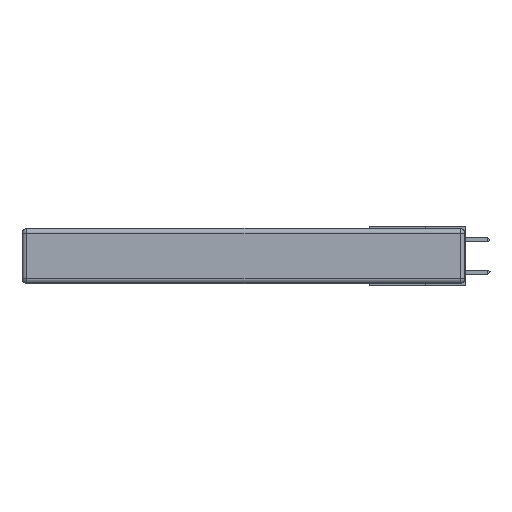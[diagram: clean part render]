
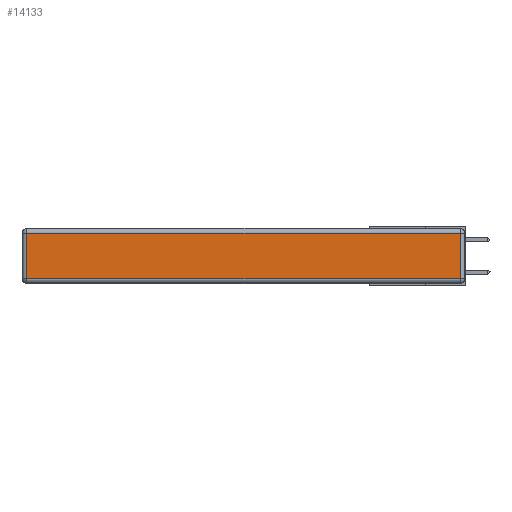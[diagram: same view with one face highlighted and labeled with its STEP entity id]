
A CAD part, left-side view. The second image highlights one B-rep face of the part: STEP entity #14133.
In plain terms, the highlighted planar face has unit normal (-1, 0, 0).
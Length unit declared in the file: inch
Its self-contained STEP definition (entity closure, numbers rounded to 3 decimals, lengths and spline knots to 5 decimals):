
#341 = DIRECTION ( 'NONE',  ( -1., 0., 0. ) ) ;
#1084 = VERTEX_POINT ( 'NONE', #22969 ) ;
#1301 = ORIENTED_EDGE ( 'NONE', *, *, #22466, .T. ) ;
#1772 = EDGE_LOOP ( 'NONE', ( #8781, #1301, #11192, #18537 ) ) ;
#1949 = PLANE ( 'NONE',  #10484 ) ;
#2592 = EDGE_CURVE ( 'NONE', #15348, #1084, #18725, .T. ) ;
#2916 = VECTOR ( 'NONE', #7739, 39.37008 ) ;
#3004 = DIRECTION ( 'NONE',  ( 0., 0., 1. ) ) ;
#3934 = CARTESIAN_POINT ( 'NONE',  ( 0., 2.72, -0.343 ) ) ;
#4475 = CARTESIAN_POINT ( 'NONE',  ( 0., 2.75, -0.03 ) ) ;
#5640 = CARTESIAN_POINT ( 'NONE',  ( 0., 0., -0.343 ) ) ;
#6208 = CARTESIAN_POINT ( 'NONE',  ( 0., 0., -0.313 ) ) ;
#7540 = VECTOR ( 'NONE', #18598, 39.37008 ) ;
#7739 = DIRECTION ( 'NONE',  ( 0., -1., 0. ) ) ;
#8554 = CARTESIAN_POINT ( 'NONE',  ( 0., 2.72, -0.03 ) ) ;
#8777 = CARTESIAN_POINT ( 'NONE',  ( 0., 0.03, -0.343 ) ) ;
#8781 = ORIENTED_EDGE ( 'NONE', *, *, #14228, .T. ) ;
#9760 = DIRECTION ( 'NONE',  ( 0., 1., 0. ) ) ;
#10146 = VERTEX_POINT ( 'NONE', #21619 ) ;
#10484 = AXIS2_PLACEMENT_3D ( 'NONE', #5640, #341, #15022 ) ;
#11192 = ORIENTED_EDGE ( 'NONE', *, *, #11920, .T. ) ;
#11920 = EDGE_CURVE ( 'NONE', #21134, #15348, #16501, .T. ) ;
#12369 = FACE_OUTER_BOUND ( 'NONE', #1772, .T. ) ;
#14116 = LINE ( 'NONE', #6208, #2916 ) ;
#14133 = ADVANCED_FACE ( 'NONE', ( #12369 ), #1949, .T. ) ;
#14228 = EDGE_CURVE ( 'NONE', #1084, #10146, #14116, .T. ) ;
#15003 = LINE ( 'NONE', #8777, #18741 ) ;
#15022 = DIRECTION ( 'NONE',  ( 0., 0., 1. ) ) ;
#15348 = VERTEX_POINT ( 'NONE', #8554 ) ;
#16501 = LINE ( 'NONE', #4475, #19656 ) ;
#18537 = ORIENTED_EDGE ( 'NONE', *, *, #2592, .T. ) ;
#18598 = DIRECTION ( 'NONE',  ( 0., 0., -1. ) ) ;
#18725 = LINE ( 'NONE', #3934, #7540 ) ;
#18741 = VECTOR ( 'NONE', #3004, 39.37008 ) ;
#19656 = VECTOR ( 'NONE', #9760, 39.37008 ) ;
#21134 = VERTEX_POINT ( 'NONE', #23417 ) ;
#21619 = CARTESIAN_POINT ( 'NONE',  ( 0., 0.03, -0.313 ) ) ;
#22466 = EDGE_CURVE ( 'NONE', #10146, #21134, #15003, .T. ) ;
#22969 = CARTESIAN_POINT ( 'NONE',  ( 0., 2.72, -0.313 ) ) ;
#23417 = CARTESIAN_POINT ( 'NONE',  ( 0., 0.03, -0.03 ) ) ;
